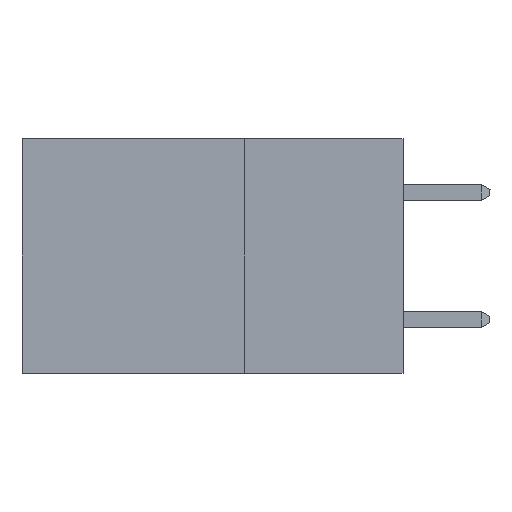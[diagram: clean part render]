
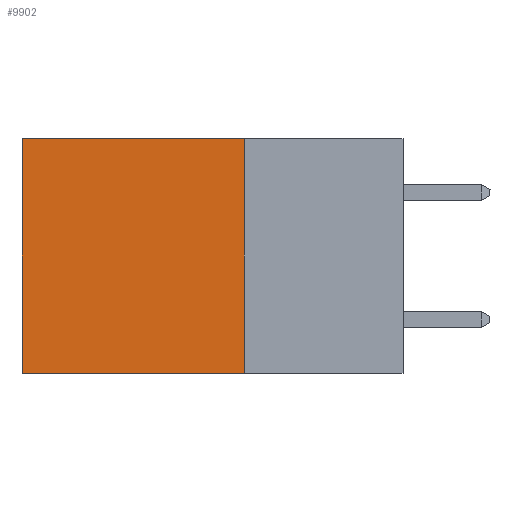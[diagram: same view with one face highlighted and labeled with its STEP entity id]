
A CAD part, left-side view. The second image highlights one B-rep face of the part: STEP entity #9902.
In plain terms, the highlighted planar face has unit normal (-1, 0, 0).
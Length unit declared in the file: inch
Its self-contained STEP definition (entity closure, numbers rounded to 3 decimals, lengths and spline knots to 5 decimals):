
#277 = DIRECTION ( 'NONE',  ( 0., 1., 0. ) ) ;
#448 = DIRECTION ( 'NONE',  ( 1., 0., 0. ) ) ;
#729 = CARTESIAN_POINT ( 'NONE',  ( 0.2875, 0.25, 0. ) ) ;
#2798 = DIRECTION ( 'NONE',  ( 0., 0., -1. ) ) ;
#2972 = VERTEX_POINT ( 'NONE', #18535 ) ;
#3931 = CARTESIAN_POINT ( 'NONE',  ( 0.2875, 0.6, 0. ) ) ;
#4076 = DIRECTION ( 'NONE',  ( 0., 1., 0. ) ) ;
#4915 = ORIENTED_EDGE ( 'NONE', *, *, #7836, .T. ) ;
#5353 = CARTESIAN_POINT ( 'NONE',  ( 0.2875, 0.25, 0. ) ) ;
#6230 = EDGE_LOOP ( 'NONE', ( #14858, #12559, #23898, #4915 ) ) ;
#6849 = AXIS2_PLACEMENT_3D ( 'NONE', #729, #448, #2798 ) ;
#7836 = EDGE_CURVE ( 'NONE', #17611, #20522, #22483, .T. ) ;
#9532 = VERTEX_POINT ( 'NONE', #17102 ) ;
#9758 = VECTOR ( 'NONE', #4076, 39.37008 ) ;
#9902 = ADVANCED_FACE ( 'NONE', ( #27332 ), #25122, .F. ) ;
#10719 = LINE ( 'NONE', #26348, #26890 ) ;
#12559 = ORIENTED_EDGE ( 'NONE', *, *, #15045, .F. ) ;
#13046 = CARTESIAN_POINT ( 'NONE',  ( 0.2875, 0.6, 0. ) ) ;
#14858 = ORIENTED_EDGE ( 'NONE', *, *, #19166, .T. ) ;
#15045 = EDGE_CURVE ( 'NONE', #2972, #9532, #19804, .T. ) ;
#15445 = CARTESIAN_POINT ( 'NONE',  ( 0.2875, 0.25, 0. ) ) ;
#15513 = LINE ( 'NONE', #13046, #20580 ) ;
#17102 = CARTESIAN_POINT ( 'NONE',  ( 0.2875, 0.6, -0.37 ) ) ;
#17611 = VERTEX_POINT ( 'NONE', #5353 ) ;
#18535 = CARTESIAN_POINT ( 'NONE',  ( 0.2875, 0.25, -0.37 ) ) ;
#19166 = EDGE_CURVE ( 'NONE', #20522, #9532, #15513, .T. ) ;
#19517 = CARTESIAN_POINT ( 'NONE',  ( 0.2875, 0.25, -0.37 ) ) ;
#19766 = DIRECTION ( 'NONE',  ( 0., 0., -1. ) ) ;
#19804 = LINE ( 'NONE', #19517, #9758 ) ;
#20522 = VERTEX_POINT ( 'NONE', #3931 ) ;
#20580 = VECTOR ( 'NONE', #19766, 39.37008 ) ;
#22483 = LINE ( 'NONE', #15445, #24455 ) ;
#23898 = ORIENTED_EDGE ( 'NONE', *, *, #24457, .F. ) ;
#24455 = VECTOR ( 'NONE', #277, 39.37008 ) ;
#24457 = EDGE_CURVE ( 'NONE', #17611, #2972, #10719, .T. ) ;
#25122 = PLANE ( 'NONE',  #6849 ) ;
#26348 = CARTESIAN_POINT ( 'NONE',  ( 0.2875, 0.25, 0. ) ) ;
#26890 = VECTOR ( 'NONE', #28561, 39.37008 ) ;
#27332 = FACE_OUTER_BOUND ( 'NONE', #6230, .T. ) ;
#28561 = DIRECTION ( 'NONE',  ( 0., 0., -1. ) ) ;
